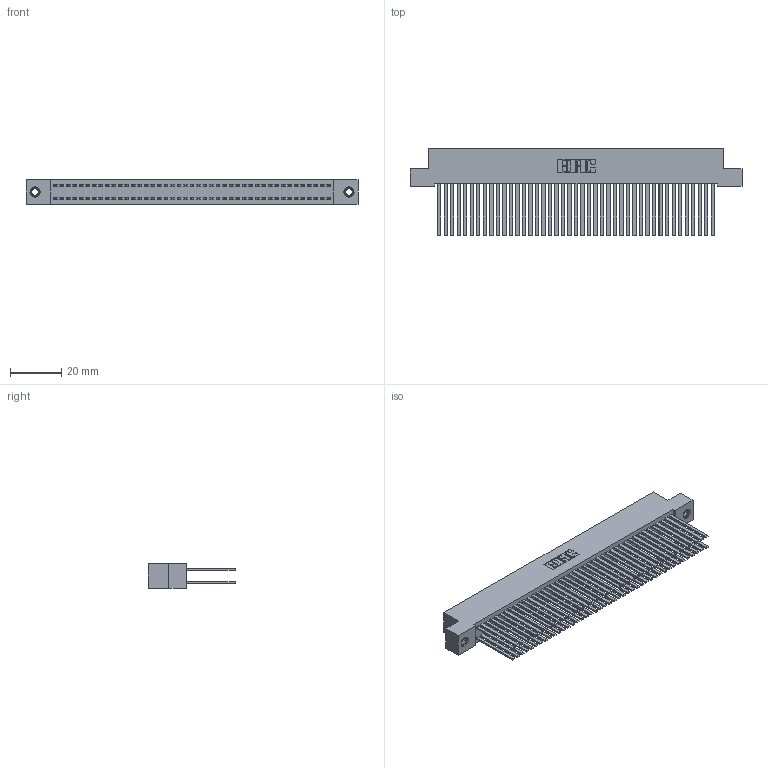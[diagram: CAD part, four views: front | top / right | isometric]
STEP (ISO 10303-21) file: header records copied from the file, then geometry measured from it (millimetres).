
FILE_DESCRIPTION (( 'STEP AP203' ), '1' );
FILE_NAME ('342-086-544-207.STEP', '2019-10-04T13:16:26', ( '' ), ( '' ), 'SwSTEP 2.0', 'SolidWorks 2016', '' );
FILE_SCHEMA (( 'CONFIG_CONTROL_DESIGN' ));
Length unit declared in the file: inch
Products named in the file (4): 342 Part_TI; 345-292-001_345-293-144; 345-250-001_345-250-005-103; 342-086-544-207
Assembly tree (89 placements, depth 2):
  342-086-544-207
    342 Part_TI
    345-292-001_345-293-144  x86
    345-250-001_345-250-005-103  x2
Bounding box: 129.54 x 34.3 x 9.4 mm (x, y, z)
Volume: 12836.8 mm3; surface area: 24284.1 mm2
Topology: 89 solids, 89 shells, 4126 faces, 12217 edges, 8022 vertices
Faces by surface type: plane 2850, cylinder 1260, cone 12, torus 4
Entity records: 28404 total; most frequent: CARTESIAN_POINT 4685, ORIENTED_EDGE 4614, DIRECTION 4029, EDGE_CURVE 2307, LINE 2163, VECTOR 2163, VERTEX_POINT 1532, AXIS2_PLACEMENT_3D 933
